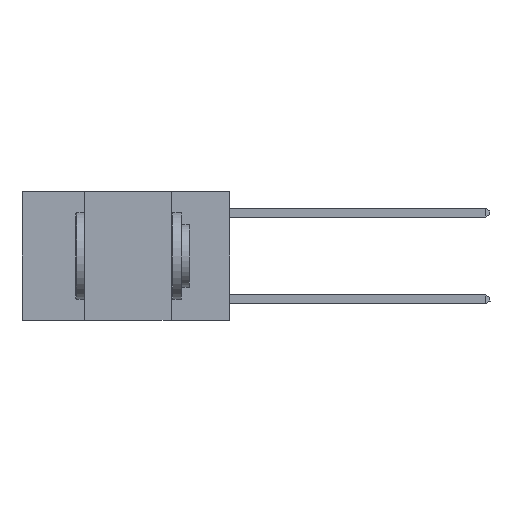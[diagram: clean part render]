
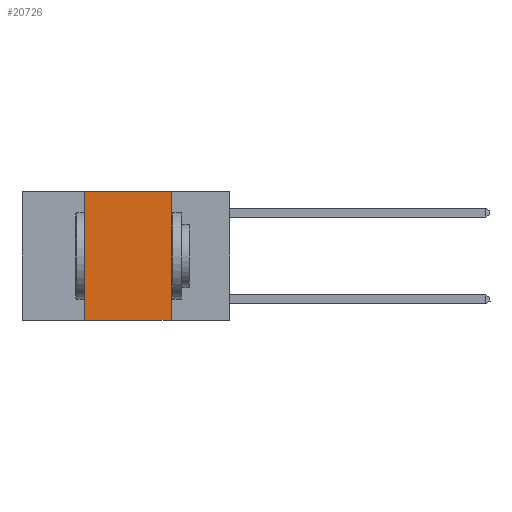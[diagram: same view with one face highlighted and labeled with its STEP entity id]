
A CAD part, left-side view. The second image highlights one B-rep face of the part: STEP entity #20726.
In plain terms, the highlighted planar face has unit normal (-1, 0, 0).
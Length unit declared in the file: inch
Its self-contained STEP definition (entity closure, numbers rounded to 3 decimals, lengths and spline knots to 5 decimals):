
#598 = CARTESIAN_POINT ( 'NONE',  ( 0., 0.17, 0. ) ) ;
#799 = ORIENTED_EDGE ( 'NONE', *, *, #10726, .F. ) ;
#1666 = CARTESIAN_POINT ( 'NONE',  ( 0., 0.6, 0. ) ) ;
#4106 = LINE ( 'NONE', #8781, #16523 ) ;
#4174 = DIRECTION ( 'NONE',  ( 0., 0., -1. ) ) ;
#4314 = ORIENTED_EDGE ( 'NONE', *, *, #12098, .T. ) ;
#5425 = CARTESIAN_POINT ( 'NONE',  ( 0., 0.42, -0.37 ) ) ;
#6452 = VERTEX_POINT ( 'NONE', #5425 ) ;
#6601 = CARTESIAN_POINT ( 'NONE',  ( 0., 0.17, -0.37 ) ) ;
#6800 = DIRECTION ( 'NONE',  ( 0., -1., 0. ) ) ;
#7987 = EDGE_CURVE ( 'NONE', #26331, #27922, #28747, .T. ) ;
#8781 = CARTESIAN_POINT ( 'NONE',  ( 0., 0.42, 0. ) ) ;
#10726 = EDGE_CURVE ( 'NONE', #29267, #26331, #20299, .T. ) ;
#11377 = LINE ( 'NONE', #24259, #23665 ) ;
#12028 = DIRECTION ( 'NONE',  ( 0., -1., 0. ) ) ;
#12098 = EDGE_CURVE ( 'NONE', #6452, #27922, #11377, .T. ) ;
#12390 = DIRECTION ( 'NONE',  ( 0., 0., -1. ) ) ;
#14168 = CARTESIAN_POINT ( 'NONE',  ( 0., 0.6, 0. ) ) ;
#15778 = FACE_OUTER_BOUND ( 'NONE', #24474, .T. ) ;
#16523 = VECTOR ( 'NONE', #25966, 39.37008 ) ;
#18992 = DIRECTION ( 'NONE',  ( 1., 0., 0. ) ) ;
#19748 = ORIENTED_EDGE ( 'NONE', *, *, #7987, .F. ) ;
#19978 = EDGE_CURVE ( 'NONE', #6452, #29267, #4106, .T. ) ;
#20299 = LINE ( 'NONE', #14168, #23724 ) ;
#20726 = ADVANCED_FACE ( 'NONE', ( #15778 ), #21332, .F. ) ;
#21318 = AXIS2_PLACEMENT_3D ( 'NONE', #1666, #18992, #4174 ) ;
#21332 = PLANE ( 'NONE',  #21318 ) ;
#22245 = VECTOR ( 'NONE', #12390, 39.37008 ) ;
#23665 = VECTOR ( 'NONE', #12028, 39.37008 ) ;
#23724 = VECTOR ( 'NONE', #6800, 39.37008 ) ;
#24259 = CARTESIAN_POINT ( 'NONE',  ( 0., 0.6, -0.37 ) ) ;
#24474 = EDGE_LOOP ( 'NONE', ( #19748, #799, #28188, #4314 ) ) ;
#24488 = CARTESIAN_POINT ( 'NONE',  ( 0., 0.17, 0. ) ) ;
#25966 = DIRECTION ( 'NONE',  ( 0., 0., 1. ) ) ;
#26331 = VERTEX_POINT ( 'NONE', #598 ) ;
#27922 = VERTEX_POINT ( 'NONE', #6601 ) ;
#28188 = ORIENTED_EDGE ( 'NONE', *, *, #19978, .F. ) ;
#28747 = LINE ( 'NONE', #24488, #22245 ) ;
#28846 = CARTESIAN_POINT ( 'NONE',  ( 0., 0.42, 0. ) ) ;
#29267 = VERTEX_POINT ( 'NONE', #28846 ) ;
